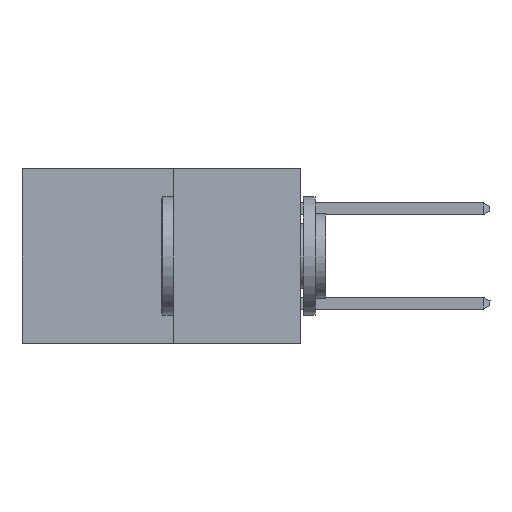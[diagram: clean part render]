
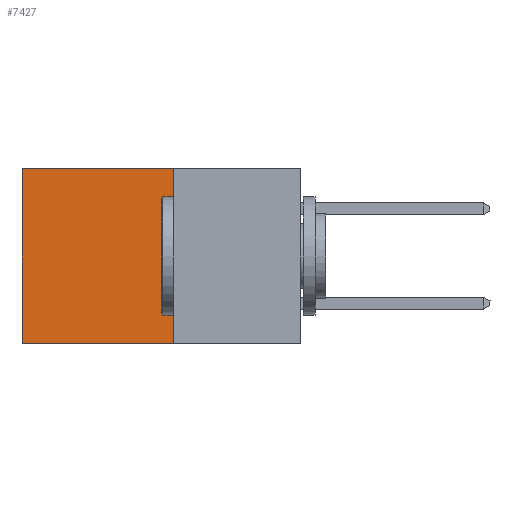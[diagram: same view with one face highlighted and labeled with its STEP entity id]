
A CAD part, left-side view. The second image highlights one B-rep face of the part: STEP entity #7427.
In plain terms, the highlighted planar face has unit normal (-1, 0, 0).
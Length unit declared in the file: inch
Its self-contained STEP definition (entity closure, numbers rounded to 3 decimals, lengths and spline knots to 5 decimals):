
#1126 = DIRECTION ( 'NONE',  ( 0., 0., -1. ) ) ;
#1309 = VECTOR ( 'NONE', #20063, 39.37008 ) ;
#1564 = CARTESIAN_POINT ( 'NONE',  ( 0.277, 0.27, -0.37 ) ) ;
#2493 = FACE_OUTER_BOUND ( 'NONE', #21164, .T. ) ;
#2767 = VERTEX_POINT ( 'NONE', #17734 ) ;
#3172 = CARTESIAN_POINT ( 'NONE',  ( 0.277, 0.59, -0.37 ) ) ;
#3460 = VERTEX_POINT ( 'NONE', #11988 ) ;
#5274 = PLANE ( 'NONE',  #7535 ) ;
#5311 = CARTESIAN_POINT ( 'NONE',  ( 0.277, 0.27, 0. ) ) ;
#6166 = EDGE_CURVE ( 'NONE', #2767, #20239, #23578, .T. ) ;
#6302 = LINE ( 'NONE', #14602, #1309 ) ;
#7427 = ADVANCED_FACE ( 'NONE', ( #2493 ), #5274, .F. ) ;
#7535 = AXIS2_PLACEMENT_3D ( 'NONE', #18189, #20016, #9055 ) ;
#8167 = EDGE_CURVE ( 'NONE', #20239, #20336, #6302, .T. ) ;
#8270 = ORIENTED_EDGE ( 'NONE', *, *, #6166, .F. ) ;
#8513 = CARTESIAN_POINT ( 'NONE',  ( 0.277, 0.27, -0.37 ) ) ;
#9055 = DIRECTION ( 'NONE',  ( 0., 0., -1. ) ) ;
#9792 = DIRECTION ( 'NONE',  ( 0., 0., -1. ) ) ;
#10367 = LINE ( 'NONE', #20714, #16381 ) ;
#10615 = EDGE_CURVE ( 'NONE', #2767, #3460, #16862, .T. ) ;
#11988 = CARTESIAN_POINT ( 'NONE',  ( 0.277, 0.59, 0. ) ) ;
#13096 = ORIENTED_EDGE ( 'NONE', *, *, #20678, .T. ) ;
#13939 = VECTOR ( 'NONE', #1126, 39.37008 ) ;
#14602 = CARTESIAN_POINT ( 'NONE',  ( 0.277, 0.27, -0.37 ) ) ;
#16381 = VECTOR ( 'NONE', #9792, 39.37008 ) ;
#16862 = LINE ( 'NONE', #5311, #21694 ) ;
#17734 = CARTESIAN_POINT ( 'NONE',  ( 0.277, 0.27, 0. ) ) ;
#18189 = CARTESIAN_POINT ( 'NONE',  ( 0.277, 0.27, -0.37 ) ) ;
#18226 = DIRECTION ( 'NONE',  ( 0., 1., 0. ) ) ;
#20016 = DIRECTION ( 'NONE',  ( 1., 0., 0. ) ) ;
#20063 = DIRECTION ( 'NONE',  ( 0., 1., 0. ) ) ;
#20124 = ORIENTED_EDGE ( 'NONE', *, *, #8167, .F. ) ;
#20239 = VERTEX_POINT ( 'NONE', #8513 ) ;
#20336 = VERTEX_POINT ( 'NONE', #3172 ) ;
#20597 = ORIENTED_EDGE ( 'NONE', *, *, #10615, .T. ) ;
#20678 = EDGE_CURVE ( 'NONE', #3460, #20336, #10367, .T. ) ;
#20714 = CARTESIAN_POINT ( 'NONE',  ( 0.277, 0.59, -0.37 ) ) ;
#21164 = EDGE_LOOP ( 'NONE', ( #13096, #20124, #8270, #20597 ) ) ;
#21694 = VECTOR ( 'NONE', #18226, 39.37008 ) ;
#23578 = LINE ( 'NONE', #1564, #13939 ) ;
